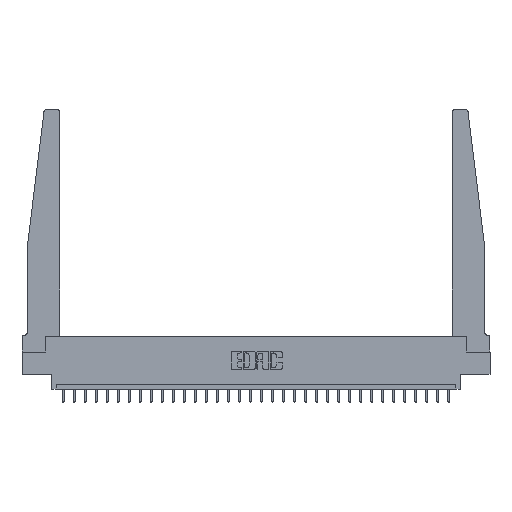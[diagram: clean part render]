
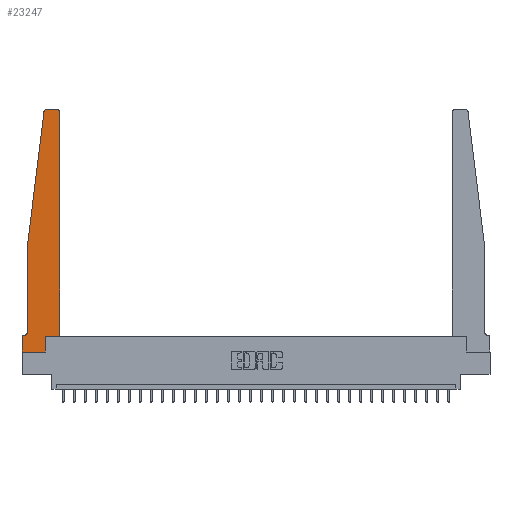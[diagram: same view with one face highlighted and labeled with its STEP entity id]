
A CAD part, top view. The second image highlights one B-rep face of the part: STEP entity #23247.
In plain terms, the highlighted planar face has unit normal (0, 0, 1).
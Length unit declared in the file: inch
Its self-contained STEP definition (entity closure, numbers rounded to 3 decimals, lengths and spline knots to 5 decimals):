
#32 = DIRECTION ( 'NONE',  ( 0., 0., 1. ) ) ;
#102 = EDGE_CURVE ( 'NONE', #20992, #24495, #18693, .T. ) ;
#240 = DIRECTION ( 'NONE',  ( 0., -1., 0. ) ) ;
#364 = VERTEX_POINT ( 'NONE', #20175 ) ;
#996 = ORIENTED_EDGE ( 'NONE', *, *, #5921, .T. ) ;
#1128 = CARTESIAN_POINT ( 'NONE',  ( 0., 0.1875, 0.37 ) ) ;
#1533 = CARTESIAN_POINT ( 'NONE',  ( 0.25, 2.75, 0.37 ) ) ;
#2000 = DIRECTION ( 'NONE',  ( 0., -1., 0. ) ) ;
#2213 = AXIS2_PLACEMENT_3D ( 'NONE', #12395, #18971, #21260 ) ;
#2552 = VERTEX_POINT ( 'NONE', #5234 ) ;
#3352 = ORIENTED_EDGE ( 'NONE', *, *, #26841, .T. ) ;
#3443 = VECTOR ( 'NONE', #27847, 39.37008 ) ;
#3605 = VECTOR ( 'NONE', #7451, 39.37008 ) ;
#3717 = CARTESIAN_POINT ( 'NONE',  ( 0., 0., 0.37 ) ) ;
#3892 = ORIENTED_EDGE ( 'NONE', *, *, #27630, .T. ) ;
#4021 = DIRECTION ( 'NONE',  ( 1., 0., 0. ) ) ;
#4295 = VERTEX_POINT ( 'NONE', #21074 ) ;
#4395 = VECTOR ( 'NONE', #240, 39.37008 ) ;
#4521 = CARTESIAN_POINT ( 'NONE',  ( 0.065, 1.25, 0.37 ) ) ;
#5234 = CARTESIAN_POINT ( 'NONE',  ( 0.065, 0.2375, 0.37 ) ) ;
#5271 = DIRECTION ( 'NONE',  ( 1., 0., 0. ) ) ;
#5921 = EDGE_CURVE ( 'NONE', #11596, #15444, #19782, .T. ) ;
#5988 = ORIENTED_EDGE ( 'NONE', *, *, #21882, .T. ) ;
#6799 = EDGE_CURVE ( 'NONE', #27996, #2552, #10193, .T. ) ;
#6971 = EDGE_CURVE ( 'NONE', #20151, #4295, #27825, .T. ) ;
#7193 = DIRECTION ( 'NONE',  ( 0., 0., -1. ) ) ;
#7282 = DIRECTION ( 'NONE',  ( 0., 0., 1. ) ) ;
#7451 = DIRECTION ( 'NONE',  ( -0.122, -0.992, 0. ) ) ;
#8343 = EDGE_LOOP ( 'NONE', ( #15097, #20607, #5988, #22806, #3352, #996, #22193, #27043, #27204, #3892, #19152, #23143 ) ) ;
#8359 = CARTESIAN_POINT ( 'NONE',  ( 0.065, 0.1875, 0.37 ) ) ;
#8368 = CIRCLE ( 'NONE', #2213, 0.03 ) ;
#8400 = CARTESIAN_POINT ( 'NONE',  ( 0.395, 2.75, 0.37 ) ) ;
#8421 = DIRECTION ( 'NONE',  ( 0., 1., 0. ) ) ;
#8824 = VECTOR ( 'NONE', #2000, 39.37008 ) ;
#10095 = CARTESIAN_POINT ( 'NONE',  ( 0.24675, 2.72367, 0.37 ) ) ;
#10193 = LINE ( 'NONE', #4521, #8824 ) ;
#10268 = EDGE_CURVE ( 'NONE', #24495, #364, #13622, .T. ) ;
#10504 = LINE ( 'NONE', #19312, #4395 ) ;
#10923 = DIRECTION ( 'NONE',  ( 1., 0., 0. ) ) ;
#11381 = CARTESIAN_POINT ( 'NONE',  ( 0.015, 0.2375, 0.37 ) ) ;
#11596 = VERTEX_POINT ( 'NONE', #24110 ) ;
#12395 = CARTESIAN_POINT ( 'NONE',  ( 0.395, 2.72, 0.37 ) ) ;
#12589 = DIRECTION ( 'NONE',  ( -1., 0., 0. ) ) ;
#12603 = VECTOR ( 'NONE', #10923, 39.37008 ) ;
#12894 = AXIS2_PLACEMENT_3D ( 'NONE', #23995, #32, #15170 ) ;
#12985 = PLANE ( 'NONE',  #12894 ) ;
#13333 = CIRCLE ( 'NONE', #18965, 0.05 ) ;
#13381 = AXIS2_PLACEMENT_3D ( 'NONE', #15942, #7282, #5271 ) ;
#13622 = LINE ( 'NONE', #27949, #3443 ) ;
#14207 = CARTESIAN_POINT ( 'NONE',  ( 0.065, 1.25, 0.37 ) ) ;
#14278 = VECTOR ( 'NONE', #4021, 39.37008 ) ;
#14371 = LINE ( 'NONE', #1533, #24921 ) ;
#15097 = ORIENTED_EDGE ( 'NONE', *, *, #25715, .T. ) ;
#15150 = LINE ( 'NONE', #14207, #3605 ) ;
#15170 = DIRECTION ( 'NONE',  ( 1., 0., 0. ) ) ;
#15444 = VERTEX_POINT ( 'NONE', #1128 ) ;
#15942 = CARTESIAN_POINT ( 'NONE',  ( 0.27653, 2.72, 0.37 ) ) ;
#15984 = LINE ( 'NONE', #23924, #12603 ) ;
#16028 = VECTOR ( 'NONE', #21135, 39.37008 ) ;
#16310 = VECTOR ( 'NONE', #8421, 39.37008 ) ;
#16423 = EDGE_CURVE ( 'NONE', #19867, #26039, #20806, .T. ) ;
#18693 = LINE ( 'NONE', #23870, #14278 ) ;
#18756 = EDGE_CURVE ( 'NONE', #15444, #20992, #10504, .T. ) ;
#18965 = AXIS2_PLACEMENT_3D ( 'NONE', #11381, #7193, #26472 ) ;
#18971 = DIRECTION ( 'NONE',  ( 0., 0., 1. ) ) ;
#19152 = ORIENTED_EDGE ( 'NONE', *, *, #6971, .T. ) ;
#19312 = CARTESIAN_POINT ( 'NONE',  ( 0., 0., 0.37 ) ) ;
#19782 = LINE ( 'NONE', #8359, #16028 ) ;
#19867 = VERTEX_POINT ( 'NONE', #22755 ) ;
#20151 = VERTEX_POINT ( 'NONE', #26261 ) ;
#20175 = CARTESIAN_POINT ( 'NONE',  ( 0.2605, 0.18, 0.37 ) ) ;
#20607 = ORIENTED_EDGE ( 'NONE', *, *, #16423, .T. ) ;
#20806 = CIRCLE ( 'NONE', #13381, 0.03 ) ;
#20992 = VERTEX_POINT ( 'NONE', #3717 ) ;
#21074 = CARTESIAN_POINT ( 'NONE',  ( 0.425, 2.72, 0.37 ) ) ;
#21075 = CARTESIAN_POINT ( 'NONE',  ( 0.2605, 0., 0.37 ) ) ;
#21135 = DIRECTION ( 'NONE',  ( -1., 0., 0. ) ) ;
#21260 = DIRECTION ( 'NONE',  ( 1., 0., 0. ) ) ;
#21882 = EDGE_CURVE ( 'NONE', #26039, #27996, #15150, .T. ) ;
#22193 = ORIENTED_EDGE ( 'NONE', *, *, #18756, .T. ) ;
#22755 = CARTESIAN_POINT ( 'NONE',  ( 0.27653, 2.75, 0.37 ) ) ;
#22806 = ORIENTED_EDGE ( 'NONE', *, *, #6799, .T. ) ;
#23143 = ORIENTED_EDGE ( 'NONE', *, *, #24433, .T. ) ;
#23247 = ADVANCED_FACE ( 'NONE', ( #25778 ), #12985, .T. ) ;
#23266 = CARTESIAN_POINT ( 'NONE',  ( 0.425, 0.18, 0.37 ) ) ;
#23870 = CARTESIAN_POINT ( 'NONE',  ( 0., 0., 0.37 ) ) ;
#23924 = CARTESIAN_POINT ( 'NONE',  ( 0.425, 0.18, 0.37 ) ) ;
#23995 = CARTESIAN_POINT ( 'NONE',  ( 0., 0.1875, 0.37 ) ) ;
#24110 = CARTESIAN_POINT ( 'NONE',  ( 0.015, 0.1875, 0.37 ) ) ;
#24433 = EDGE_CURVE ( 'NONE', #4295, #24571, #8368, .T. ) ;
#24495 = VERTEX_POINT ( 'NONE', #21075 ) ;
#24571 = VERTEX_POINT ( 'NONE', #8400 ) ;
#24921 = VECTOR ( 'NONE', #12589, 39.37008 ) ;
#25715 = EDGE_CURVE ( 'NONE', #24571, #19867, #14371, .T. ) ;
#25778 = FACE_OUTER_BOUND ( 'NONE', #8343, .T. ) ;
#26039 = VERTEX_POINT ( 'NONE', #10095 ) ;
#26261 = CARTESIAN_POINT ( 'NONE',  ( 0.425, 0.18, 0.37 ) ) ;
#26472 = DIRECTION ( 'NONE',  ( -1., 0., 0. ) ) ;
#26841 = EDGE_CURVE ( 'NONE', #2552, #11596, #13333, .T. ) ;
#27043 = ORIENTED_EDGE ( 'NONE', *, *, #102, .T. ) ;
#27204 = ORIENTED_EDGE ( 'NONE', *, *, #10268, .T. ) ;
#27288 = CARTESIAN_POINT ( 'NONE',  ( 0.065, 1.25, 0.37 ) ) ;
#27630 = EDGE_CURVE ( 'NONE', #364, #20151, #15984, .T. ) ;
#27825 = LINE ( 'NONE', #23266, #16310 ) ;
#27847 = DIRECTION ( 'NONE',  ( 0., 1., 0. ) ) ;
#27949 = CARTESIAN_POINT ( 'NONE',  ( 0.2605, 0.18, 0.37 ) ) ;
#27996 = VERTEX_POINT ( 'NONE', #27288 ) ;
